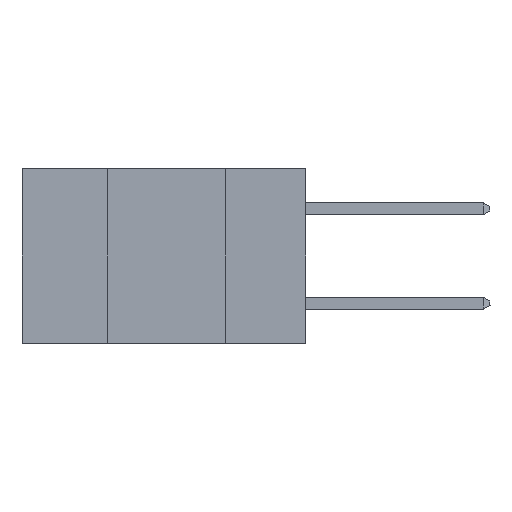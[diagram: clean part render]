
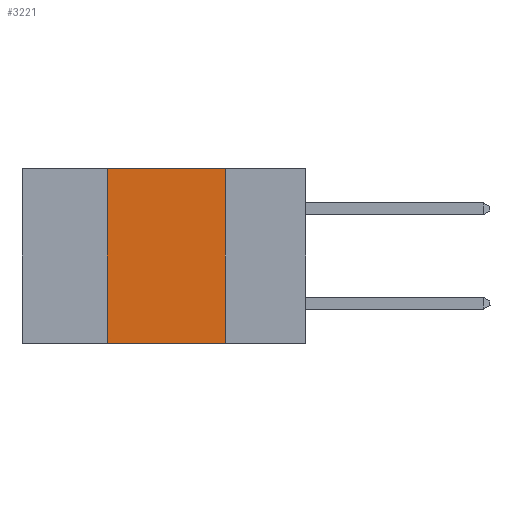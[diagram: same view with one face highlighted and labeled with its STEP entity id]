
A CAD part, left-side view. The second image highlights one B-rep face of the part: STEP entity #3221.
In plain terms, the highlighted planar face has unit normal (-1, 0, 0).
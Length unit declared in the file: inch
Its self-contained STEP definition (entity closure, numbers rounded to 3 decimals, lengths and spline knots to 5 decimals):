
#348 = DIRECTION ( 'NONE',  ( 0., 0., 1. ) ) ;
#1444 = DIRECTION ( 'NONE',  ( 0., 0., -1. ) ) ;
#1730 = ORIENTED_EDGE ( 'NONE', *, *, #14719, .F. ) ;
#2228 = VERTEX_POINT ( 'NONE', #19628 ) ;
#2244 = VERTEX_POINT ( 'NONE', #10067 ) ;
#2294 = VECTOR ( 'NONE', #1444, 39.37008 ) ;
#2556 = VECTOR ( 'NONE', #18937, 39.37008 ) ;
#3221 = ADVANCED_FACE ( 'NONE', ( #29830 ), #20822, .F. ) ;
#4929 = ORIENTED_EDGE ( 'NONE', *, *, #16239, .F. ) ;
#6004 = CARTESIAN_POINT ( 'NONE',  ( 0., 0.42, -0.37 ) ) ;
#6247 = DIRECTION ( 'NONE',  ( 0., -1., 0. ) ) ;
#6875 = ORIENTED_EDGE ( 'NONE', *, *, #12975, .F. ) ;
#7562 = VECTOR ( 'NONE', #348, 39.37008 ) ;
#9391 = ORIENTED_EDGE ( 'NONE', *, *, #11547, .T. ) ;
#10067 = CARTESIAN_POINT ( 'NONE',  ( 0., 0.42, 0. ) ) ;
#11547 = EDGE_CURVE ( 'NONE', #27114, #22549, #27298, .T. ) ;
#12821 = VECTOR ( 'NONE', #6247, 39.37008 ) ;
#12975 = EDGE_CURVE ( 'NONE', #2244, #2228, #13562, .T. ) ;
#13562 = LINE ( 'NONE', #29449, #12821 ) ;
#14719 = EDGE_CURVE ( 'NONE', #27114, #2244, #26088, .T. ) ;
#16239 = EDGE_CURVE ( 'NONE', #2228, #22549, #20996, .T. ) ;
#18937 = DIRECTION ( 'NONE',  ( 0., -1., 0. ) ) ;
#19628 = CARTESIAN_POINT ( 'NONE',  ( 0., 0.17, 0. ) ) ;
#19742 = AXIS2_PLACEMENT_3D ( 'NONE', #20665, #20866, #20903 ) ;
#20665 = CARTESIAN_POINT ( 'NONE',  ( 0., 0.6, 0. ) ) ;
#20822 = PLANE ( 'NONE',  #19742 ) ;
#20866 = DIRECTION ( 'NONE',  ( 1., 0., 0. ) ) ;
#20903 = DIRECTION ( 'NONE',  ( 0., 0., -1. ) ) ;
#20996 = LINE ( 'NONE', #29315, #2294 ) ;
#21238 = CARTESIAN_POINT ( 'NONE',  ( 0., 0.17, -0.37 ) ) ;
#22549 = VERTEX_POINT ( 'NONE', #21238 ) ;
#22671 = EDGE_LOOP ( 'NONE', ( #4929, #6875, #1730, #9391 ) ) ;
#23658 = CARTESIAN_POINT ( 'NONE',  ( 0., 0.42, 0. ) ) ;
#25747 = CARTESIAN_POINT ( 'NONE',  ( 0., 0.6, -0.37 ) ) ;
#26088 = LINE ( 'NONE', #23658, #7562 ) ;
#27114 = VERTEX_POINT ( 'NONE', #6004 ) ;
#27298 = LINE ( 'NONE', #25747, #2556 ) ;
#29315 = CARTESIAN_POINT ( 'NONE',  ( 0., 0.17, 0. ) ) ;
#29449 = CARTESIAN_POINT ( 'NONE',  ( 0., 0.6, 0. ) ) ;
#29830 = FACE_OUTER_BOUND ( 'NONE', #22671, .T. ) ;
